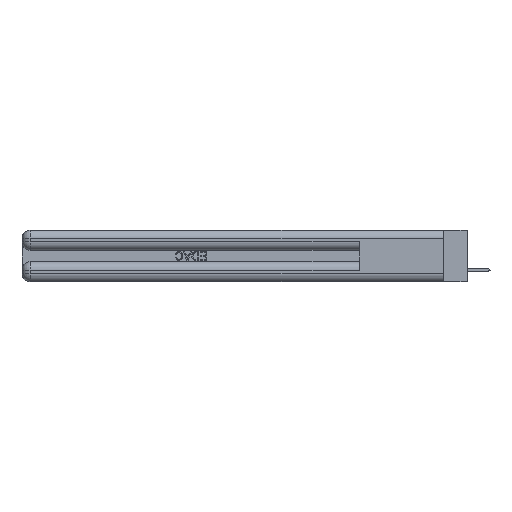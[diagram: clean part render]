
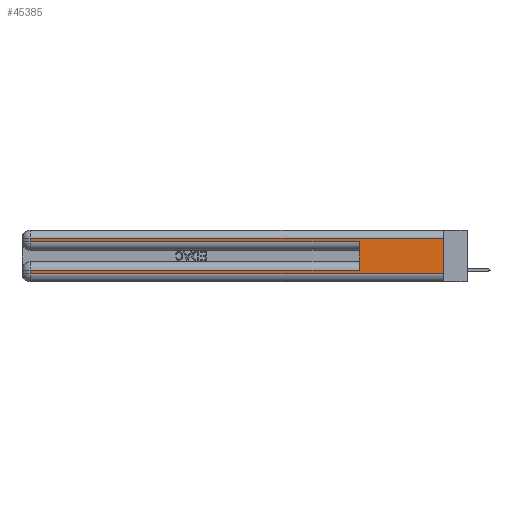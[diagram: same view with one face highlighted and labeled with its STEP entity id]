
A CAD part, left-side view. The second image highlights one B-rep face of the part: STEP entity #45385.
In plain terms, the highlighted planar face has unit normal (-1, 0, 0).
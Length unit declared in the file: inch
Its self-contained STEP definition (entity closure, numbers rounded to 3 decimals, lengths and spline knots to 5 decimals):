
#1216 = CARTESIAN_POINT ( 'NONE',  ( 0., 0., 0.06 ) ) ;
#2535 = DIRECTION ( 'NONE',  ( 0., -1., 0. ) ) ;
#2876 = EDGE_CURVE ( 'NONE', #33588, #33720, #29932, .T. ) ;
#4472 = DIRECTION ( 'NONE',  ( 0., 0., -1. ) ) ;
#4806 = ORIENTED_EDGE ( 'NONE', *, *, #34971, .F. ) ;
#6354 = CARTESIAN_POINT ( 'NONE',  ( 0., 0., 0.37 ) ) ;
#7290 = EDGE_CURVE ( 'NONE', #20674, #26585, #24113, .T. ) ;
#8116 = CARTESIAN_POINT ( 'NONE',  ( 0., 2.94, 0.085 ) ) ;
#8243 = CARTESIAN_POINT ( 'NONE',  ( 0., 0., 0.37 ) ) ;
#9208 = CARTESIAN_POINT ( 'NONE',  ( 0., 0., 0.31 ) ) ;
#9853 = DIRECTION ( 'NONE',  ( 1., 0., 0. ) ) ;
#10066 = DIRECTION ( 'NONE',  ( 0., 1., 0. ) ) ;
#10181 = LINE ( 'NONE', #41358, #37850 ) ;
#11850 = CARTESIAN_POINT ( 'NONE',  ( 0., 0.6, 0.145 ) ) ;
#15334 = DIRECTION ( 'NONE',  ( 0., 0., 1. ) ) ;
#16701 = EDGE_CURVE ( 'NONE', #21763, #32320, #38837, .T. ) ;
#17035 = ORIENTED_EDGE ( 'NONE', *, *, #16701, .T. ) ;
#17517 = LINE ( 'NONE', #45868, #25188 ) ;
#18129 = LINE ( 'NONE', #11850, #45214 ) ;
#19693 = EDGE_CURVE ( 'NONE', #33720, #23330, #17517, .T. ) ;
#20674 = VERTEX_POINT ( 'NONE', #27556 ) ;
#21068 = CARTESIAN_POINT ( 'NONE',  ( 0., 0., 0.31 ) ) ;
#21216 = CARTESIAN_POINT ( 'NONE',  ( 0., 2.94, 0.31 ) ) ;
#21353 = PLANE ( 'NONE',  #22515 ) ;
#21763 = VERTEX_POINT ( 'NONE', #25360 ) ;
#21775 = ORIENTED_EDGE ( 'NONE', *, *, #19693, .T. ) ;
#22515 = AXIS2_PLACEMENT_3D ( 'NONE', #6354, #9853, #24513 ) ;
#23312 = DIRECTION ( 'NONE',  ( 0., 0., -1. ) ) ;
#23330 = VERTEX_POINT ( 'NONE', #28821 ) ;
#24113 = LINE ( 'NONE', #32185, #41188 ) ;
#24513 = DIRECTION ( 'NONE',  ( 0., 0., -1. ) ) ;
#24744 = LINE ( 'NONE', #8243, #30621 ) ;
#24990 = EDGE_CURVE ( 'NONE', #32320, #20674, #10181, .T. ) ;
#25188 = VECTOR ( 'NONE', #23312, 39.37008 ) ;
#25360 = CARTESIAN_POINT ( 'NONE',  ( 0., 0.6, 0.085 ) ) ;
#26349 = DIRECTION ( 'NONE',  ( 0., -1., 0. ) ) ;
#26562 = DIRECTION ( 'NONE',  ( 0., 0., -1. ) ) ;
#26585 = VERTEX_POINT ( 'NONE', #1216 ) ;
#27001 = EDGE_CURVE ( 'NONE', #33588, #26585, #24744, .T. ) ;
#27037 = ORIENTED_EDGE ( 'NONE', *, *, #24990, .T. ) ;
#27556 = CARTESIAN_POINT ( 'NONE',  ( 0., 2.94, 0.06 ) ) ;
#28338 = CARTESIAN_POINT ( 'NONE',  ( 0., 0., 0.085 ) ) ;
#28821 = CARTESIAN_POINT ( 'NONE',  ( 0., 2.94, 0.285 ) ) ;
#28872 = VERTEX_POINT ( 'NONE', #38613 ) ;
#29932 = LINE ( 'NONE', #21068, #39323 ) ;
#29961 = LINE ( 'NONE', #37279, #48758 ) ;
#30621 = VECTOR ( 'NONE', #26562, 39.37008 ) ;
#32185 = CARTESIAN_POINT ( 'NONE',  ( 0., 0., 0.06 ) ) ;
#32230 = EDGE_LOOP ( 'NONE', ( #38564, #42584, #21775, #36846, #4806, #17035, #27037, #42514 ) ) ;
#32320 = VERTEX_POINT ( 'NONE', #8116 ) ;
#33329 = FACE_OUTER_BOUND ( 'NONE', #32230, .T. ) ;
#33588 = VERTEX_POINT ( 'NONE', #9208 ) ;
#33720 = VERTEX_POINT ( 'NONE', #21216 ) ;
#34905 = EDGE_CURVE ( 'NONE', #23330, #28872, #29961, .T. ) ;
#34971 = EDGE_CURVE ( 'NONE', #21763, #28872, #18129, .T. ) ;
#36846 = ORIENTED_EDGE ( 'NONE', *, *, #34905, .T. ) ;
#37279 = CARTESIAN_POINT ( 'NONE',  ( 0., 0., 0.285 ) ) ;
#37850 = VECTOR ( 'NONE', #4472, 39.37008 ) ;
#38564 = ORIENTED_EDGE ( 'NONE', *, *, #27001, .F. ) ;
#38613 = CARTESIAN_POINT ( 'NONE',  ( 0., 0.6, 0.285 ) ) ;
#38837 = LINE ( 'NONE', #28338, #39426 ) ;
#39323 = VECTOR ( 'NONE', #10066, 39.37008 ) ;
#39426 = VECTOR ( 'NONE', #46749, 39.37008 ) ;
#41188 = VECTOR ( 'NONE', #2535, 39.37008 ) ;
#41358 = CARTESIAN_POINT ( 'NONE',  ( 0., 2.94, 0.37 ) ) ;
#42514 = ORIENTED_EDGE ( 'NONE', *, *, #7290, .T. ) ;
#42584 = ORIENTED_EDGE ( 'NONE', *, *, #2876, .T. ) ;
#45214 = VECTOR ( 'NONE', #15334, 39.37008 ) ;
#45385 = ADVANCED_FACE ( 'NONE', ( #33329 ), #21353, .F. ) ;
#45868 = CARTESIAN_POINT ( 'NONE',  ( 0., 2.94, 0.37 ) ) ;
#46749 = DIRECTION ( 'NONE',  ( 0., 1., 0. ) ) ;
#48758 = VECTOR ( 'NONE', #26349, 39.37008 ) ;
